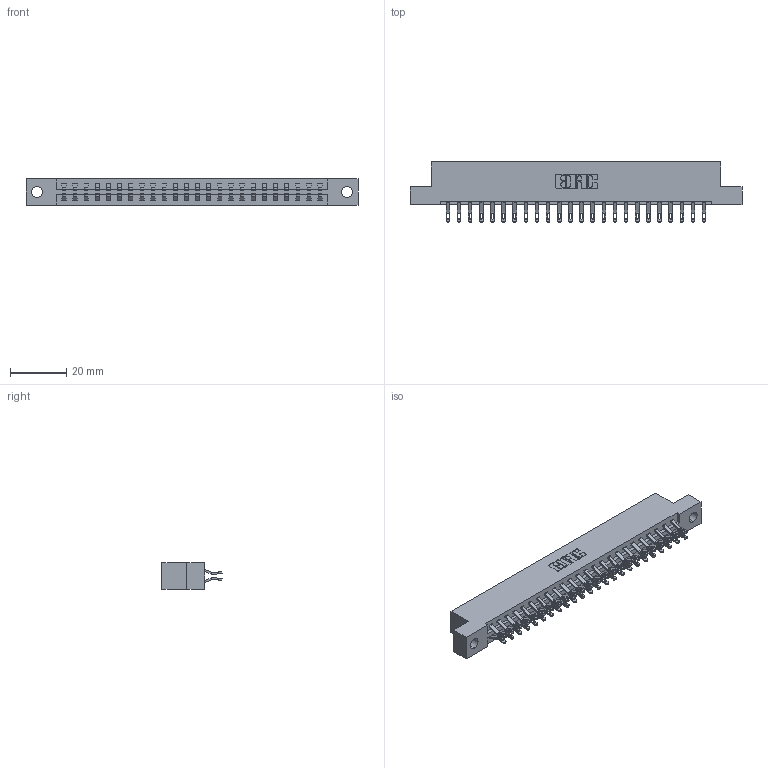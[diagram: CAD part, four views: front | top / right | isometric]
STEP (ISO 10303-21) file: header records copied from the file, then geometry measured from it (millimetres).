
FILE_DESCRIPTION (( 'STEP AP203' ), '1' );
FILE_NAME ('387-048-555-204.STEP', '2019-10-18T10:19:40', ( '' ), ( '' ), 'SwSTEP 2.0', 'SolidWorks 2016', '' );
FILE_SCHEMA (( 'CONFIG_CONTROL_DESIGN' ));
Length unit declared in the file: inch
Products named in the file (3): 345-292-001_555 Tail; 337 Part_Flush Mounting Lugs - 0.156 Dia-TH; 387-048-555-204
Assembly tree (49 placements, depth 2):
  387-048-555-204
    337 Part_Flush Mounting Lugs - 0.156 Dia-TH
    345-292-001_555 Tail  x48
Bounding box: 118.11 x 21.47 x 9.4 mm (x, y, z)
Volume: 12259.1 mm3; surface area: 14006.2 mm2
Topology: 49 solids, 49 shells, 2994 faces, 9383 edges, 6254 vertices
Faces by surface type: plane 1798, cylinder 1196
Entity records: 21265 total; most frequent: CARTESIAN_POINT 3632, ORIENTED_EDGE 3538, DIRECTION 3093, EDGE_CURVE 1769, LINE 1621, VECTOR 1621, VERTEX_POINT 1178, AXIS2_PLACEMENT_3D 736
